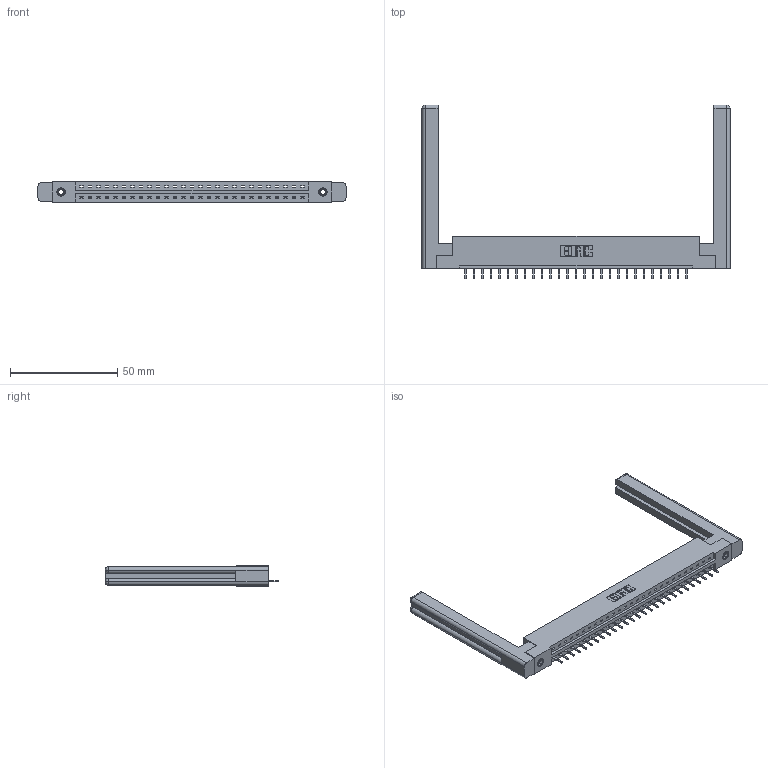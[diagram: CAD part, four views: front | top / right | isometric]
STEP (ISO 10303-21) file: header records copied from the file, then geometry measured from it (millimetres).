
FILE_DESCRIPTION (( 'STEP AP203' ), '1' );
FILE_NAME ('337-027-520-158.STEP', '2019-09-30T19:21:59', ( '' ), ( '' ), 'SwSTEP 2.0', 'SolidWorks 2016', '' );
FILE_SCHEMA (( 'CONFIG_CONTROL_DESIGN' ));
Length unit declared in the file: inch
Products named in the file (5): 337-027-520-158; 307-220-058; 345-250-001_345-250-001-102; 337 Part_Flush Mounting Lugs - 0.156 Dia-TI; 345-292-001_345-293-120
Assembly tree (32 placements, depth 2):
  337-027-520-158
    337 Part_Flush Mounting Lugs - 0.156 Dia-TI
    345-292-001_345-293-120  x27
    345-250-001_345-250-001-102  x2
    307-220-058  x2
Bounding box: 143.61 x 81.11 x 9.4 mm (x, y, z)
Volume: 21822.8 mm3; surface area: 19999.8 mm2
Topology: 32 solids, 32 shells, 2038 faces, 5957 edges, 3886 vertices
Faces by surface type: plane 1450, cylinder 564, cone 12, torus 12
Entity records: 24758 total; most frequent: CARTESIAN_POINT 4322, ORIENTED_EDGE 4212, DIRECTION 3676, EDGE_CURVE 2106, VECTOR 1926, LINE 1926, VERTEX_POINT 1394, AXIS2_PLACEMENT_3D 875
